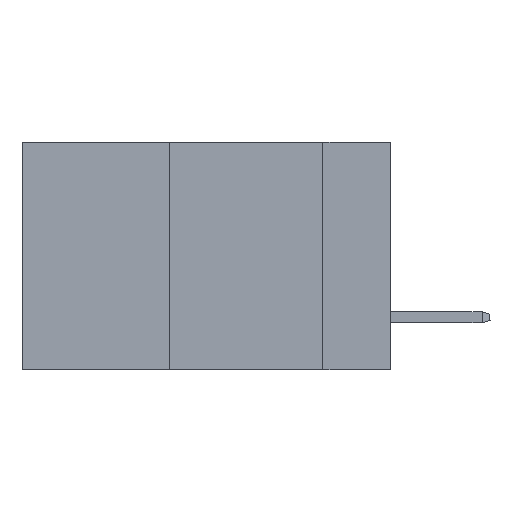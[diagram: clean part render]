
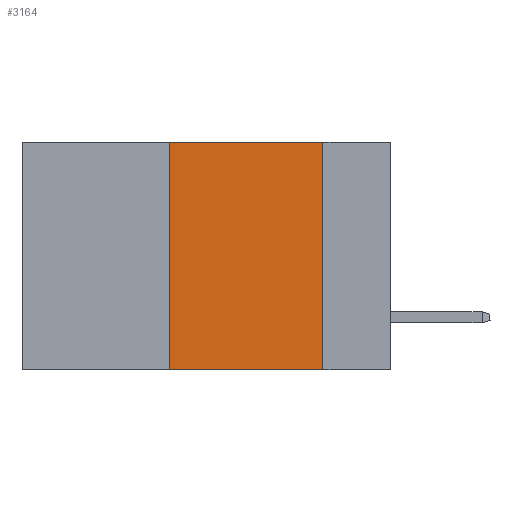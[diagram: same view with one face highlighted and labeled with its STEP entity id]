
A CAD part, left-side view. The second image highlights one B-rep face of the part: STEP entity #3164.
In plain terms, the highlighted planar face has unit normal (-1, 0, 0).
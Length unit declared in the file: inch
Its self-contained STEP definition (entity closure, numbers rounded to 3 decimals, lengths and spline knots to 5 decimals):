
#665 = DIRECTION ( 'NONE',  ( 0., 0., 1. ) ) ;
#685 = DIRECTION ( 'NONE',  ( 1., 0., 0. ) ) ;
#1104 = VECTOR ( 'NONE', #3663, 39.37008 ) ;
#1304 = DIRECTION ( 'NONE',  ( 0., 0., -1. ) ) ;
#2261 = DIRECTION ( 'NONE',  ( 0., -1., 0. ) ) ;
#2302 = CARTESIAN_POINT ( 'NONE',  ( 0., 0.36, -0.37 ) ) ;
#2328 = CARTESIAN_POINT ( 'NONE',  ( 0., 0.6, 0. ) ) ;
#3064 = VECTOR ( 'NONE', #2261, 39.37008 ) ;
#3164 = ADVANCED_FACE ( 'NONE', ( #10769 ), #4684, .F. ) ;
#3310 = ORIENTED_EDGE ( 'NONE', *, *, #7376, .F. ) ;
#3620 = CARTESIAN_POINT ( 'NONE',  ( 0., 0.6, -0.37 ) ) ;
#3663 = DIRECTION ( 'NONE',  ( 0., -1., 0. ) ) ;
#4004 = DIRECTION ( 'NONE',  ( 0., 0., -1. ) ) ;
#4591 = CARTESIAN_POINT ( 'NONE',  ( 0., 0.11, 0. ) ) ;
#4684 = PLANE ( 'NONE',  #9087 ) ;
#4874 = ORIENTED_EDGE ( 'NONE', *, *, #7324, .F. ) ;
#4891 = LINE ( 'NONE', #3620, #1104 ) ;
#5410 = VERTEX_POINT ( 'NONE', #2302 ) ;
#5705 = EDGE_CURVE ( 'NONE', #7247, #7742, #5892, .T. ) ;
#5835 = EDGE_LOOP ( 'NONE', ( #10278, #3310, #4874, #7146 ) ) ;
#5892 = LINE ( 'NONE', #10389, #8652 ) ;
#5979 = CARTESIAN_POINT ( 'NONE',  ( 0., 0.11, -0.37 ) ) ;
#6543 = CARTESIAN_POINT ( 'NONE',  ( 0., 0.36, 0. ) ) ;
#6867 = VERTEX_POINT ( 'NONE', #10021 ) ;
#7146 = ORIENTED_EDGE ( 'NONE', *, *, #8732, .T. ) ;
#7243 = CARTESIAN_POINT ( 'NONE',  ( 0., 0.6, 0. ) ) ;
#7247 = VERTEX_POINT ( 'NONE', #4591 ) ;
#7324 = EDGE_CURVE ( 'NONE', #5410, #6867, #9271, .T. ) ;
#7376 = EDGE_CURVE ( 'NONE', #6867, #7247, #8473, .T. ) ;
#7742 = VERTEX_POINT ( 'NONE', #5979 ) ;
#8350 = VECTOR ( 'NONE', #665, 39.37008 ) ;
#8473 = LINE ( 'NONE', #2328, #3064 ) ;
#8652 = VECTOR ( 'NONE', #1304, 39.37008 ) ;
#8732 = EDGE_CURVE ( 'NONE', #5410, #7742, #4891, .T. ) ;
#9087 = AXIS2_PLACEMENT_3D ( 'NONE', #7243, #685, #4004 ) ;
#9271 = LINE ( 'NONE', #6543, #8350 ) ;
#10021 = CARTESIAN_POINT ( 'NONE',  ( 0., 0.36, 0. ) ) ;
#10278 = ORIENTED_EDGE ( 'NONE', *, *, #5705, .F. ) ;
#10389 = CARTESIAN_POINT ( 'NONE',  ( 0., 0.11, 0. ) ) ;
#10769 = FACE_OUTER_BOUND ( 'NONE', #5835, .T. ) ;
